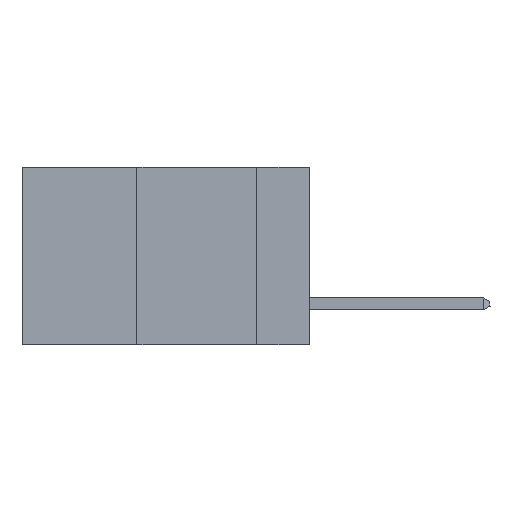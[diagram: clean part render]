
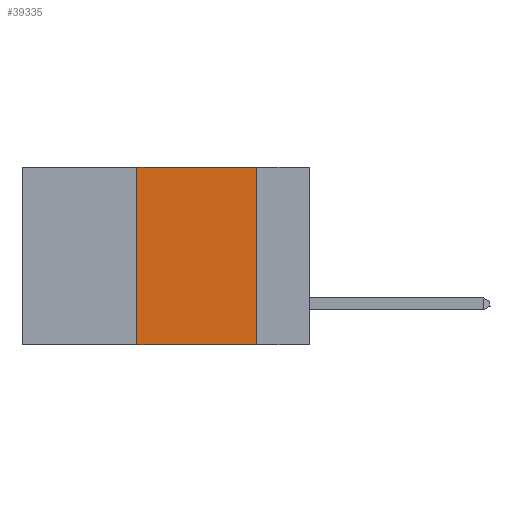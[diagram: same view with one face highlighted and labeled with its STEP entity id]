
A CAD part, left-side view. The second image highlights one B-rep face of the part: STEP entity #39335.
In plain terms, the highlighted planar face has unit normal (-1, 0, 0).
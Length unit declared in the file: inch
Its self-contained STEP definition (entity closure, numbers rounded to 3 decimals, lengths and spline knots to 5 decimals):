
#392 = EDGE_CURVE ( 'NONE', #1980, #10571, #17876, .T. ) ;
#1980 = VERTEX_POINT ( 'NONE', #23703 ) ;
#1983 = FACE_OUTER_BOUND ( 'NONE', #12499, .T. ) ;
#3619 = CARTESIAN_POINT ( 'NONE',  ( 0., 0.6, 0. ) ) ;
#4254 = VERTEX_POINT ( 'NONE', #22889 ) ;
#4314 = VERTEX_POINT ( 'NONE', #11902 ) ;
#5411 = DIRECTION ( 'NONE',  ( 1., 0., 0. ) ) ;
#5556 = VECTOR ( 'NONE', #11774, 39.37008 ) ;
#5773 = DIRECTION ( 'NONE',  ( 0., 0., -1. ) ) ;
#5799 = ORIENTED_EDGE ( 'NONE', *, *, #20941, .T. ) ;
#6521 = VECTOR ( 'NONE', #12691, 39.37008 ) ;
#10571 = VERTEX_POINT ( 'NONE', #19305 ) ;
#11774 = DIRECTION ( 'NONE',  ( 0., -1., 0. ) ) ;
#11902 = CARTESIAN_POINT ( 'NONE',  ( 0., 0.36, -0.37 ) ) ;
#12499 = EDGE_LOOP ( 'NONE', ( #15094, #48291, #37414, #5799 ) ) ;
#12691 = DIRECTION ( 'NONE',  ( 0., -1., 0. ) ) ;
#12887 = CARTESIAN_POINT ( 'NONE',  ( 0., 0.6, -0.37 ) ) ;
#15094 = ORIENTED_EDGE ( 'NONE', *, *, #392, .F. ) ;
#16295 = CARTESIAN_POINT ( 'NONE',  ( 0., 0.11, 0. ) ) ;
#17876 = LINE ( 'NONE', #16295, #37333 ) ;
#18268 = EDGE_CURVE ( 'NONE', #4254, #1980, #34914, .T. ) ;
#19305 = CARTESIAN_POINT ( 'NONE',  ( 0., 0.11, -0.37 ) ) ;
#20066 = EDGE_CURVE ( 'NONE', #4314, #4254, #26836, .T. ) ;
#20846 = AXIS2_PLACEMENT_3D ( 'NONE', #36369, #5411, #5773 ) ;
#20941 = EDGE_CURVE ( 'NONE', #4314, #10571, #24168, .T. ) ;
#22889 = CARTESIAN_POINT ( 'NONE',  ( 0., 0.36, 0. ) ) ;
#23703 = CARTESIAN_POINT ( 'NONE',  ( 0., 0.11, 0. ) ) ;
#24168 = LINE ( 'NONE', #12887, #6521 ) ;
#24353 = DIRECTION ( 'NONE',  ( 0., 0., 1. ) ) ;
#26836 = LINE ( 'NONE', #47494, #35769 ) ;
#34914 = LINE ( 'NONE', #3619, #5556 ) ;
#35240 = DIRECTION ( 'NONE',  ( 0., 0., -1. ) ) ;
#35769 = VECTOR ( 'NONE', #24353, 39.37008 ) ;
#36369 = CARTESIAN_POINT ( 'NONE',  ( 0., 0.6, 0. ) ) ;
#37333 = VECTOR ( 'NONE', #35240, 39.37008 ) ;
#37414 = ORIENTED_EDGE ( 'NONE', *, *, #20066, .F. ) ;
#39335 = ADVANCED_FACE ( 'NONE', ( #1983 ), #46600, .F. ) ;
#46600 = PLANE ( 'NONE',  #20846 ) ;
#47494 = CARTESIAN_POINT ( 'NONE',  ( 0., 0.36, 0. ) ) ;
#48291 = ORIENTED_EDGE ( 'NONE', *, *, #18268, .F. ) ;
